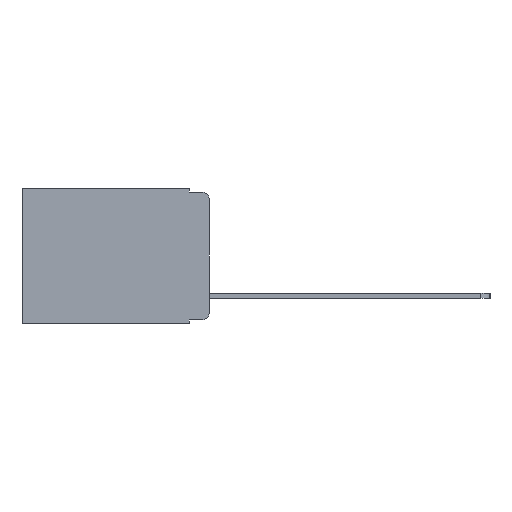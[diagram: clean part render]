
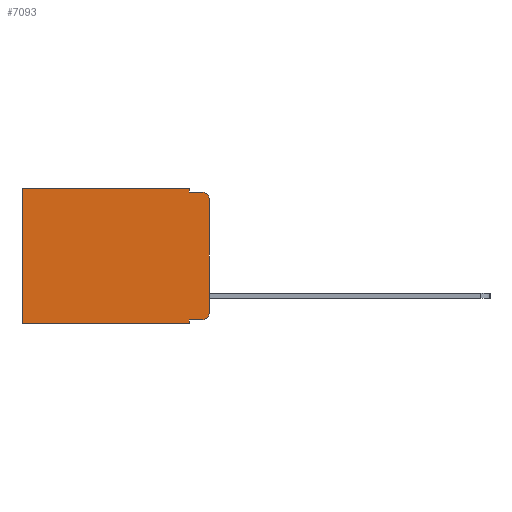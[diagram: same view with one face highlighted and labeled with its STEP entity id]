
A CAD part, left-side view. The second image highlights one B-rep face of the part: STEP entity #7093.
In plain terms, the highlighted planar face has unit normal (-1, 0, 0).
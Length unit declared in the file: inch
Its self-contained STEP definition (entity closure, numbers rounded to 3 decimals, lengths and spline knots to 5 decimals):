
#583 = ORIENTED_EDGE ( 'NONE', *, *, #9982, .T. ) ;
#717 = EDGE_CURVE ( 'NONE', #7417, #1437, #2678, .T. ) ;
#846 = CARTESIAN_POINT ( 'NONE',  ( 0.298, 0.051, -0.01 ) ) ;
#896 = DIRECTION ( 'NONE',  ( 0., 0., -1. ) ) ;
#941 = DIRECTION ( 'NONE',  ( 0., 0., -1. ) ) ;
#950 = ORIENTED_EDGE ( 'NONE', *, *, #10096, .T. ) ;
#1281 = VERTEX_POINT ( 'NONE', #8366 ) ;
#1418 = ORIENTED_EDGE ( 'NONE', *, *, #9965, .F. ) ;
#1437 = VERTEX_POINT ( 'NONE', #3648 ) ;
#1744 = AXIS2_PLACEMENT_3D ( 'NONE', #10057, #3588, #9299 ) ;
#1798 = CARTESIAN_POINT ( 'NONE',  ( 0.298, 0.051, -0.343 ) ) ;
#2037 = VECTOR ( 'NONE', #896, 39.37008 ) ;
#2215 = VERTEX_POINT ( 'NONE', #6444 ) ;
#2652 = CIRCLE ( 'NONE', #5302, 0.02 ) ;
#2654 = CARTESIAN_POINT ( 'NONE',  ( 0.298, 0., 0. ) ) ;
#2656 = PLANE ( 'NONE',  #1744 ) ;
#2678 = LINE ( 'NONE', #3015, #7174 ) ;
#2763 = VERTEX_POINT ( 'NONE', #10954 ) ;
#2826 = CARTESIAN_POINT ( 'NONE',  ( 0.298, 0.02, -0.03 ) ) ;
#2867 = CARTESIAN_POINT ( 'NONE',  ( 0.298, 0.051, 0. ) ) ;
#2885 = CARTESIAN_POINT ( 'NONE',  ( 0.298, 0.051, -0.333 ) ) ;
#2932 = ORIENTED_EDGE ( 'NONE', *, *, #6876, .F. ) ;
#2991 = CARTESIAN_POINT ( 'NONE',  ( 0.298, 0.02, -0.313 ) ) ;
#3015 = CARTESIAN_POINT ( 'NONE',  ( 0.298, 0., 0. ) ) ;
#3528 = VECTOR ( 'NONE', #10928, 39.37008 ) ;
#3588 = DIRECTION ( 'NONE',  ( 1., 0., 0. ) ) ;
#3648 = CARTESIAN_POINT ( 'NONE',  ( 0.298, 0.473, 0. ) ) ;
#3735 = DIRECTION ( 'NONE',  ( 0., 0., -1. ) ) ;
#3830 = LINE ( 'NONE', #4109, #10051 ) ;
#3887 = DIRECTION ( 'NONE',  ( 0., 0., -1. ) ) ;
#4109 = CARTESIAN_POINT ( 'NONE',  ( 0.298, 0., -0.343 ) ) ;
#4184 = VECTOR ( 'NONE', #10274, 39.37008 ) ;
#4287 = VERTEX_POINT ( 'NONE', #6132 ) ;
#4589 = CARTESIAN_POINT ( 'NONE',  ( 0.298, 0.02, -0.333 ) ) ;
#4756 = ORIENTED_EDGE ( 'NONE', *, *, #9996, .F. ) ;
#4806 = ORIENTED_EDGE ( 'NONE', *, *, #9999, .T. ) ;
#5173 = AXIS2_PLACEMENT_3D ( 'NONE', #2991, #8816, #3887 ) ;
#5302 = AXIS2_PLACEMENT_3D ( 'NONE', #2826, #8676, #3735 ) ;
#5309 = ORIENTED_EDGE ( 'NONE', *, *, #9963, .T. ) ;
#5689 = DIRECTION ( 'NONE',  ( 0., 1., 0. ) ) ;
#6132 = CARTESIAN_POINT ( 'NONE',  ( 0.298, 0.473, -0.343 ) ) ;
#6245 = ORIENTED_EDGE ( 'NONE', *, *, #717, .T. ) ;
#6346 = LINE ( 'NONE', #7863, #6636 ) ;
#6444 = CARTESIAN_POINT ( 'NONE',  ( 0.298, 0.02, -0.01 ) ) ;
#6636 = VECTOR ( 'NONE', #7941, 39.37008 ) ;
#6754 = VERTEX_POINT ( 'NONE', #4589 ) ;
#6876 = EDGE_CURVE ( 'NONE', #10873, #4287, #3830, .T. ) ;
#6996 = ORIENTED_EDGE ( 'NONE', *, *, #9910, .F. ) ;
#7093 = ADVANCED_FACE ( 'NONE', ( #8099 ), #2656, .F. ) ;
#7174 = VECTOR ( 'NONE', #5689, 39.37008 ) ;
#7417 = VERTEX_POINT ( 'NONE', #10309 ) ;
#7863 = CARTESIAN_POINT ( 'NONE',  ( 0.298, 0.051, -0.333 ) ) ;
#7903 = CARTESIAN_POINT ( 'NONE',  ( 0.298, 0.051, 0. ) ) ;
#7941 = DIRECTION ( 'NONE',  ( 0., -1., 0. ) ) ;
#8099 = FACE_OUTER_BOUND ( 'NONE', #9394, .T. ) ;
#8325 = VECTOR ( 'NONE', #941, 39.37008 ) ;
#8366 = CARTESIAN_POINT ( 'NONE',  ( 0.298, 0.051, -0.01 ) ) ;
#8572 = LINE ( 'NONE', #9457, #4184 ) ;
#8676 = DIRECTION ( 'NONE',  ( -1., 0., 0. ) ) ;
#8816 = DIRECTION ( 'NONE',  ( -1., 0., 0. ) ) ;
#8819 = VECTOR ( 'NONE', #11016, 39.37008 ) ;
#9049 = LINE ( 'NONE', #7903, #2037 ) ;
#9299 = DIRECTION ( 'NONE',  ( 0., 0., -1. ) ) ;
#9394 = EDGE_LOOP ( 'NONE', ( #6996, #5309, #1418, #10150, #6245, #583, #2932, #4756, #4806, #950 ) ) ;
#9407 = VERTEX_POINT ( 'NONE', #2885 ) ;
#9457 = CARTESIAN_POINT ( 'NONE',  ( 0.298, 0.473, 0. ) ) ;
#9764 = LINE ( 'NONE', #2654, #3528 ) ;
#9818 = DIRECTION ( 'NONE',  ( 0., 1., 0. ) ) ;
#9910 = EDGE_CURVE ( 'NONE', #2763, #10584, #9764, .T. ) ;
#9963 = EDGE_CURVE ( 'NONE', #2763, #2215, #2652, .T. ) ;
#9965 = EDGE_CURVE ( 'NONE', #1281, #2215, #10926, .T. ) ;
#9980 = EDGE_CURVE ( 'NONE', #7417, #1281, #9049, .T. ) ;
#9982 = EDGE_CURVE ( 'NONE', #1437, #4287, #8572, .T. ) ;
#9996 = EDGE_CURVE ( 'NONE', #9407, #10873, #10415, .T. ) ;
#9999 = EDGE_CURVE ( 'NONE', #9407, #6754, #6346, .T. ) ;
#10051 = VECTOR ( 'NONE', #9818, 39.37008 ) ;
#10057 = CARTESIAN_POINT ( 'NONE',  ( 0.298, 0., 0. ) ) ;
#10096 = EDGE_CURVE ( 'NONE', #6754, #10584, #10148, .T. ) ;
#10148 = CIRCLE ( 'NONE', #5173, 0.02 ) ;
#10150 = ORIENTED_EDGE ( 'NONE', *, *, #9980, .F. ) ;
#10274 = DIRECTION ( 'NONE',  ( 0., 0., -1. ) ) ;
#10309 = CARTESIAN_POINT ( 'NONE',  ( 0.298, 0.051, 0. ) ) ;
#10415 = LINE ( 'NONE', #2867, #8325 ) ;
#10478 = CARTESIAN_POINT ( 'NONE',  ( 0.298, 0., -0.313 ) ) ;
#10584 = VERTEX_POINT ( 'NONE', #10478 ) ;
#10873 = VERTEX_POINT ( 'NONE', #1798 ) ;
#10926 = LINE ( 'NONE', #846, #8819 ) ;
#10928 = DIRECTION ( 'NONE',  ( 0., 0., -1. ) ) ;
#10954 = CARTESIAN_POINT ( 'NONE',  ( 0.298, 0., -0.03 ) ) ;
#11016 = DIRECTION ( 'NONE',  ( 0., -1., 0. ) ) ;
